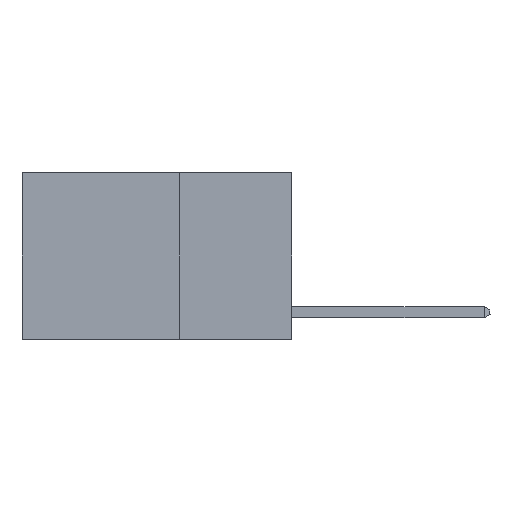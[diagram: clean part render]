
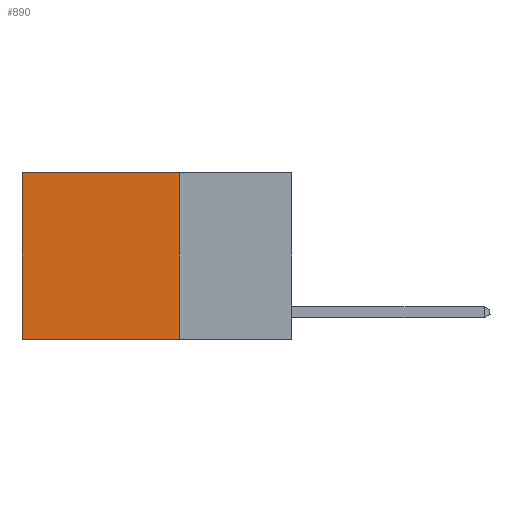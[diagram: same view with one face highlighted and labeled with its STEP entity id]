
A CAD part, left-side view. The second image highlights one B-rep face of the part: STEP entity #890.
In plain terms, the highlighted planar face has unit normal (-1, 0, 0).
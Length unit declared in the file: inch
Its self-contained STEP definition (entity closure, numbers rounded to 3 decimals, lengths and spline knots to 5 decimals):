
#169 = EDGE_CURVE ( 'NONE', #9216, #16152, #24344, .T. ) ;
#890 = ADVANCED_FACE ( 'NONE', ( #15404 ), #25642, .F. ) ;
#1281 = VECTOR ( 'NONE', #8859, 39.37008 ) ;
#2229 = EDGE_LOOP ( 'NONE', ( #21202, #13382, #12309, #22904 ) ) ;
#3926 = VECTOR ( 'NONE', #16168, 39.37008 ) ;
#4080 = CARTESIAN_POINT ( 'NONE',  ( 0.2625, 0.25, 0. ) ) ;
#4323 = CARTESIAN_POINT ( 'NONE',  ( 0.2625, 0.25, 0. ) ) ;
#4481 = DIRECTION ( 'NONE',  ( 1., 0., 0. ) ) ;
#5010 = CARTESIAN_POINT ( 'NONE',  ( 0.2625, 0.25, -0.37 ) ) ;
#5448 = VECTOR ( 'NONE', #22965, 39.37008 ) ;
#6109 = LINE ( 'NONE', #25407, #1281 ) ;
#6820 = AXIS2_PLACEMENT_3D ( 'NONE', #18694, #4481, #21065 ) ;
#8859 = DIRECTION ( 'NONE',  ( 0., 0., -1. ) ) ;
#9216 = VERTEX_POINT ( 'NONE', #4080 ) ;
#9264 = VERTEX_POINT ( 'NONE', #18782 ) ;
#12102 = CARTESIAN_POINT ( 'NONE',  ( 0.2625, 0.6, 0. ) ) ;
#12309 = ORIENTED_EDGE ( 'NONE', *, *, #28900, .F. ) ;
#13281 = CARTESIAN_POINT ( 'NONE',  ( 0.2625, 0.25, -0.37 ) ) ;
#13382 = ORIENTED_EDGE ( 'NONE', *, *, #17098, .F. ) ;
#15404 = FACE_OUTER_BOUND ( 'NONE', #2229, .T. ) ;
#16152 = VERTEX_POINT ( 'NONE', #12102 ) ;
#16168 = DIRECTION ( 'NONE',  ( 0., 1., 0. ) ) ;
#17098 = EDGE_CURVE ( 'NONE', #21614, #9264, #21750, .T. ) ;
#18694 = CARTESIAN_POINT ( 'NONE',  ( 0.2625, 0.25, 0. ) ) ;
#18782 = CARTESIAN_POINT ( 'NONE',  ( 0.2625, 0.6, -0.37 ) ) ;
#21065 = DIRECTION ( 'NONE',  ( 0., 0., -1. ) ) ;
#21202 = ORIENTED_EDGE ( 'NONE', *, *, #27670, .T. ) ;
#21614 = VERTEX_POINT ( 'NONE', #5010 ) ;
#21750 = LINE ( 'NONE', #13281, #28063 ) ;
#22904 = ORIENTED_EDGE ( 'NONE', *, *, #169, .T. ) ;
#22965 = DIRECTION ( 'NONE',  ( 0., 0., -1. ) ) ;
#23618 = LINE ( 'NONE', #29986, #5448 ) ;
#24344 = LINE ( 'NONE', #4323, #3926 ) ;
#25076 = DIRECTION ( 'NONE',  ( 0., 1., 0. ) ) ;
#25407 = CARTESIAN_POINT ( 'NONE',  ( 0.2625, 0.25, 0. ) ) ;
#25642 = PLANE ( 'NONE',  #6820 ) ;
#27670 = EDGE_CURVE ( 'NONE', #16152, #9264, #23618, .T. ) ;
#28063 = VECTOR ( 'NONE', #25076, 39.37008 ) ;
#28900 = EDGE_CURVE ( 'NONE', #9216, #21614, #6109, .T. ) ;
#29986 = CARTESIAN_POINT ( 'NONE',  ( 0.2625, 0.6, 0. ) ) ;
